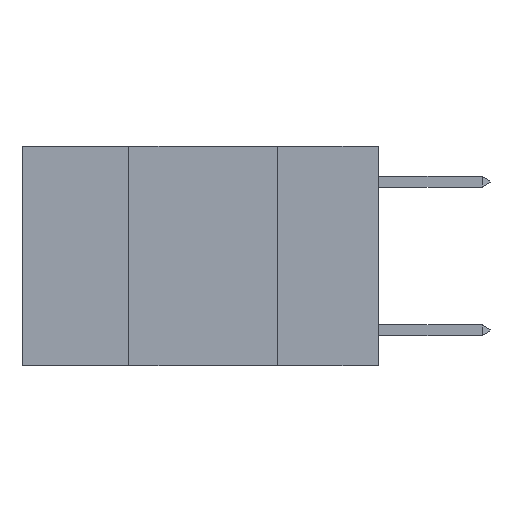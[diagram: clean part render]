
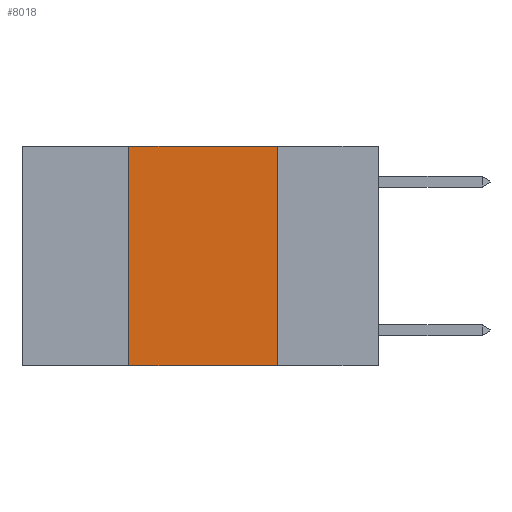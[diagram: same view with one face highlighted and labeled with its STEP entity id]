
A CAD part, left-side view. The second image highlights one B-rep face of the part: STEP entity #8018.
In plain terms, the highlighted planar face has unit normal (-1, 0, 0).
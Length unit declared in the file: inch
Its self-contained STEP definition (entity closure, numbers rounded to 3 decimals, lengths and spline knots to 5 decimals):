
#534 = EDGE_CURVE ( 'NONE', #14905, #1071, #10521, .T. ) ;
#774 = FACE_OUTER_BOUND ( 'NONE', #16247, .T. ) ;
#869 = DIRECTION ( 'NONE',  ( 0., -1., 0. ) ) ;
#1071 = VERTEX_POINT ( 'NONE', #7637 ) ;
#3294 = VERTEX_POINT ( 'NONE', #11938 ) ;
#3810 = VECTOR ( 'NONE', #13721, 39.37008 ) ;
#4518 = VECTOR ( 'NONE', #869, 39.37008 ) ;
#4574 = CARTESIAN_POINT ( 'NONE',  ( 0., 0.42, 0. ) ) ;
#4703 = VECTOR ( 'NONE', #5066, 39.37008 ) ;
#4760 = EDGE_CURVE ( 'NONE', #3294, #14905, #13045, .T. ) ;
#5066 = DIRECTION ( 'NONE',  ( 0., -1., 0. ) ) ;
#5926 = AXIS2_PLACEMENT_3D ( 'NONE', #18813, #10017, #8008 ) ;
#7637 = CARTESIAN_POINT ( 'NONE',  ( 0., 0.17, 0. ) ) ;
#8008 = DIRECTION ( 'NONE',  ( 0., 0., -1. ) ) ;
#8018 = ADVANCED_FACE ( 'NONE', ( #774 ), #18688, .F. ) ;
#9307 = DIRECTION ( 'NONE',  ( 0., 0., -1. ) ) ;
#10017 = DIRECTION ( 'NONE',  ( 1., 0., 0. ) ) ;
#10521 = LINE ( 'NONE', #16210, #4703 ) ;
#11616 = EDGE_CURVE ( 'NONE', #1071, #18924, #18443, .T. ) ;
#11938 = CARTESIAN_POINT ( 'NONE',  ( 0., 0.42, -0.37 ) ) ;
#13045 = LINE ( 'NONE', #4574, #3810 ) ;
#13721 = DIRECTION ( 'NONE',  ( 0., 0., 1. ) ) ;
#13794 = ORIENTED_EDGE ( 'NONE', *, *, #11616, .F. ) ;
#14905 = VERTEX_POINT ( 'NONE', #15330 ) ;
#15106 = LINE ( 'NONE', #22463, #4518 ) ;
#15330 = CARTESIAN_POINT ( 'NONE',  ( 0., 0.42, 0. ) ) ;
#16210 = CARTESIAN_POINT ( 'NONE',  ( 0., 0.6, 0. ) ) ;
#16247 = EDGE_LOOP ( 'NONE', ( #13794, #20916, #16603, #21975 ) ) ;
#16571 = CARTESIAN_POINT ( 'NONE',  ( 0., 0.17, -0.37 ) ) ;
#16603 = ORIENTED_EDGE ( 'NONE', *, *, #4760, .F. ) ;
#16835 = VECTOR ( 'NONE', #9307, 39.37008 ) ;
#18217 = EDGE_CURVE ( 'NONE', #3294, #18924, #15106, .T. ) ;
#18443 = LINE ( 'NONE', #22119, #16835 ) ;
#18688 = PLANE ( 'NONE',  #5926 ) ;
#18813 = CARTESIAN_POINT ( 'NONE',  ( 0., 0.6, 0. ) ) ;
#18924 = VERTEX_POINT ( 'NONE', #16571 ) ;
#20916 = ORIENTED_EDGE ( 'NONE', *, *, #534, .F. ) ;
#21975 = ORIENTED_EDGE ( 'NONE', *, *, #18217, .T. ) ;
#22119 = CARTESIAN_POINT ( 'NONE',  ( 0., 0.17, 0. ) ) ;
#22463 = CARTESIAN_POINT ( 'NONE',  ( 0., 0.6, -0.37 ) ) ;
